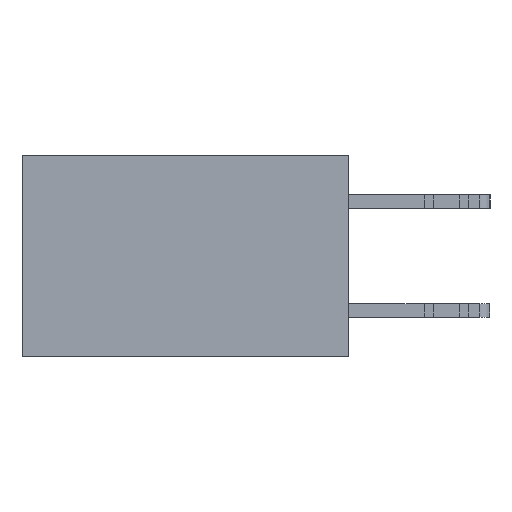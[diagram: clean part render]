
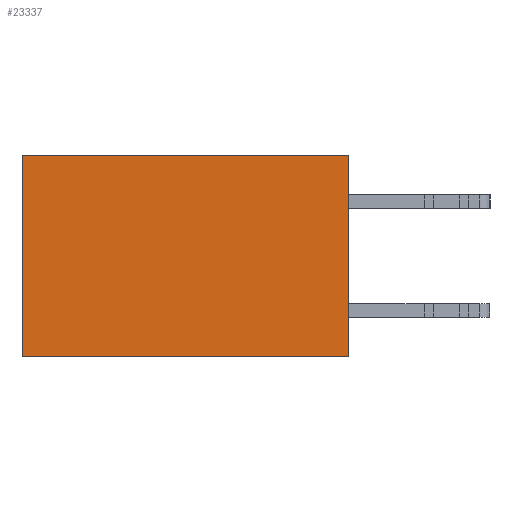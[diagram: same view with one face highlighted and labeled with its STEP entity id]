
A CAD part, left-side view. The second image highlights one B-rep face of the part: STEP entity #23337.
In plain terms, the highlighted planar face has unit normal (-1, 0, 0).
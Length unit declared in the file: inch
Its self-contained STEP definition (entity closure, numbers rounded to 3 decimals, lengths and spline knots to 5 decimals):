
#62 = CARTESIAN_POINT ( 'NONE',  ( 0.2615, 0., -0.37 ) ) ;
#688 = VERTEX_POINT ( 'NONE', #26318 ) ;
#1142 = EDGE_CURVE ( 'NONE', #10264, #2310, #17521, .T. ) ;
#2091 = DIRECTION ( 'NONE',  ( 0., 0., -1. ) ) ;
#2240 = VECTOR ( 'NONE', #2091, 39.37008 ) ;
#2310 = VERTEX_POINT ( 'NONE', #14673 ) ;
#2792 = ORIENTED_EDGE ( 'NONE', *, *, #22584, .T. ) ;
#3395 = PLANE ( 'NONE',  #12127 ) ;
#3783 = EDGE_LOOP ( 'NONE', ( #13522, #7311, #19842, #2792 ) ) ;
#5597 = VECTOR ( 'NONE', #20358, 39.37008 ) ;
#5881 = CARTESIAN_POINT ( 'NONE',  ( 0.2615, 0., 0. ) ) ;
#6688 = EDGE_CURVE ( 'NONE', #688, #2310, #26151, .T. ) ;
#7311 = ORIENTED_EDGE ( 'NONE', *, *, #6688, .F. ) ;
#7358 = DIRECTION ( 'NONE',  ( 0., 0., -1. ) ) ;
#7623 = CARTESIAN_POINT ( 'NONE',  ( 0.2615, 0., -0.37 ) ) ;
#7716 = CARTESIAN_POINT ( 'NONE',  ( 0.2615, 0., -0.37 ) ) ;
#9454 = LINE ( 'NONE', #5881, #5597 ) ;
#10264 = VERTEX_POINT ( 'NONE', #16532 ) ;
#11822 = CARTESIAN_POINT ( 'NONE',  ( 0.2615, 0.6, -0.37 ) ) ;
#11855 = EDGE_CURVE ( 'NONE', #15272, #688, #20633, .T. ) ;
#12127 = AXIS2_PLACEMENT_3D ( 'NONE', #7716, #22063, #24220 ) ;
#13413 = FACE_OUTER_BOUND ( 'NONE', #3783, .T. ) ;
#13522 = ORIENTED_EDGE ( 'NONE', *, *, #1142, .T. ) ;
#13815 = VECTOR ( 'NONE', #15889, 39.37008 ) ;
#14673 = CARTESIAN_POINT ( 'NONE',  ( 0.2615, 0.6, -0.37 ) ) ;
#15272 = VERTEX_POINT ( 'NONE', #26686 ) ;
#15889 = DIRECTION ( 'NONE',  ( 0., 1., 0. ) ) ;
#16532 = CARTESIAN_POINT ( 'NONE',  ( 0.2615, 0.6, 0. ) ) ;
#17521 = LINE ( 'NONE', #11822, #19510 ) ;
#19510 = VECTOR ( 'NONE', #7358, 39.37008 ) ;
#19842 = ORIENTED_EDGE ( 'NONE', *, *, #11855, .F. ) ;
#20358 = DIRECTION ( 'NONE',  ( 0., 1., 0. ) ) ;
#20633 = LINE ( 'NONE', #62, #2240 ) ;
#22063 = DIRECTION ( 'NONE',  ( 1., 0., 0. ) ) ;
#22584 = EDGE_CURVE ( 'NONE', #15272, #10264, #9454, .T. ) ;
#23337 = ADVANCED_FACE ( 'NONE', ( #13413 ), #3395, .F. ) ;
#24220 = DIRECTION ( 'NONE',  ( 0., 0., -1. ) ) ;
#26151 = LINE ( 'NONE', #7623, #13815 ) ;
#26318 = CARTESIAN_POINT ( 'NONE',  ( 0.2615, 0., -0.37 ) ) ;
#26686 = CARTESIAN_POINT ( 'NONE',  ( 0.2615, 0., 0. ) ) ;
